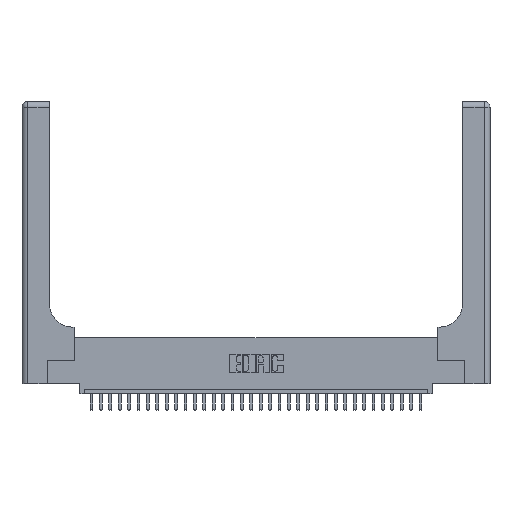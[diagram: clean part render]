
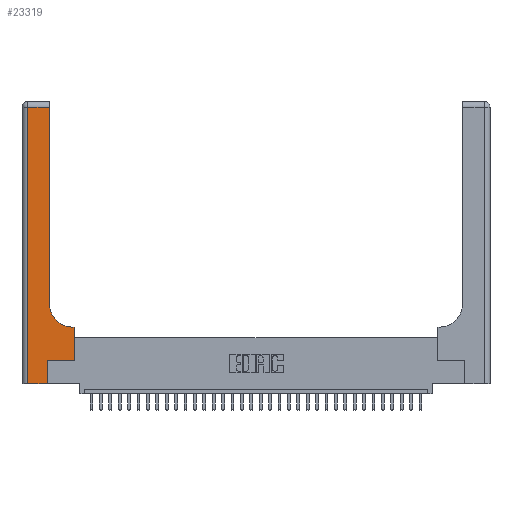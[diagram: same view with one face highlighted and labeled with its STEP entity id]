
A CAD part, top view. The second image highlights one B-rep face of the part: STEP entity #23319.
In plain terms, the highlighted planar face has unit normal (0, 0, 1).
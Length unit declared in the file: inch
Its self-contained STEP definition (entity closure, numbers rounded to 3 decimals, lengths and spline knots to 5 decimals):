
#301 = CARTESIAN_POINT ( 'NONE',  ( 0.06, 0., 0.37 ) ) ;
#767 = VECTOR ( 'NONE', #25287, 39.37008 ) ;
#1210 = CARTESIAN_POINT ( 'NONE',  ( 0.269, 0., 0.37 ) ) ;
#1386 = ORIENTED_EDGE ( 'NONE', *, *, #9491, .T. ) ;
#1639 = ORIENTED_EDGE ( 'NONE', *, *, #12392, .T. ) ;
#2786 = VERTEX_POINT ( 'NONE', #31323 ) ;
#3208 = CARTESIAN_POINT ( 'NONE',  ( 0.269, 0.25, 0.37 ) ) ;
#3319 = EDGE_CURVE ( 'NONE', #9044, #29370, #5518, .T. ) ;
#3731 = ORIENTED_EDGE ( 'NONE', *, *, #3319, .T. ) ;
#4740 = CARTESIAN_POINT ( 'NONE',  ( 0.5585, 0.6, 0.37 ) ) ;
#4770 = DIRECTION ( 'NONE',  ( 0., -1., 0. ) ) ;
#5312 = EDGE_CURVE ( 'NONE', #5352, #24309, #23494, .T. ) ;
#5352 = VERTEX_POINT ( 'NONE', #1210 ) ;
#5518 = LINE ( 'NONE', #20309, #29640 ) ;
#5809 = DIRECTION ( 'NONE',  ( 1., 0., 0. ) ) ;
#6129 = LINE ( 'NONE', #3208, #24587 ) ;
#6761 = VECTOR ( 'NONE', #26643, 39.37008 ) ;
#7242 = CARTESIAN_POINT ( 'NONE',  ( 0.5585, 0.25, 0.37 ) ) ;
#7351 = DIRECTION ( 'NONE',  ( 0., 0., -1. ) ) ;
#7523 = CARTESIAN_POINT ( 'NONE',  ( 0.269, 0.25, 0.37 ) ) ;
#7587 = EDGE_CURVE ( 'NONE', #28732, #2786, #20780, .T. ) ;
#7592 = LINE ( 'NONE', #20160, #767 ) ;
#8343 = ORIENTED_EDGE ( 'NONE', *, *, #32940, .T. ) ;
#8374 = CARTESIAN_POINT ( 'NONE',  ( 0., 3., 0.37 ) ) ;
#8383 = VERTEX_POINT ( 'NONE', #4740 ) ;
#8498 = ORIENTED_EDGE ( 'NONE', *, *, #11908, .T. ) ;
#8546 = CARTESIAN_POINT ( 'NONE',  ( 0.2915, 0.6, 0.37 ) ) ;
#8710 = DIRECTION ( 'NONE',  ( -1., 0., 0. ) ) ;
#9044 = VERTEX_POINT ( 'NONE', #19348 ) ;
#9491 = EDGE_CURVE ( 'NONE', #29370, #5352, #13828, .T. ) ;
#9790 = FACE_OUTER_BOUND ( 'NONE', #30020, .T. ) ;
#10191 = VECTOR ( 'NONE', #12410, 39.37008 ) ;
#10947 = DIRECTION ( 'NONE',  ( -1., 0., 0. ) ) ;
#11908 = EDGE_CURVE ( 'NONE', #2786, #16672, #7592, .T. ) ;
#12227 = LINE ( 'NONE', #16707, #14230 ) ;
#12392 = EDGE_CURVE ( 'NONE', #8383, #28732, #12775, .T. ) ;
#12410 = DIRECTION ( 'NONE',  ( 0., 1., 0. ) ) ;
#12775 = LINE ( 'NONE', #8546, #6761 ) ;
#12814 = DIRECTION ( 'NONE',  ( 0., 1., 0. ) ) ;
#12843 = CARTESIAN_POINT ( 'NONE',  ( 0.2915, 2.94, 0.37 ) ) ;
#13432 = DIRECTION ( 'NONE',  ( 0., 0., -1. ) ) ;
#13496 = CARTESIAN_POINT ( 'NONE',  ( 0., 0., 0.37 ) ) ;
#13828 = LINE ( 'NONE', #13496, #30327 ) ;
#14230 = VECTOR ( 'NONE', #8710, 39.37008 ) ;
#16614 = EDGE_CURVE ( 'NONE', #30853, #8383, #32746, .T. ) ;
#16672 = VERTEX_POINT ( 'NONE', #12843 ) ;
#16707 = CARTESIAN_POINT ( 'NONE',  ( 0., 2.94, 0.37 ) ) ;
#17613 = DIRECTION ( 'NONE',  ( 1., 0., 0. ) ) ;
#19348 = CARTESIAN_POINT ( 'NONE',  ( 0.06, 2.94, 0.37 ) ) ;
#20160 = CARTESIAN_POINT ( 'NONE',  ( 0.2915, 3., 0.37 ) ) ;
#20309 = CARTESIAN_POINT ( 'NONE',  ( 0.06, 3., 0.37 ) ) ;
#20780 = CIRCLE ( 'NONE', #29693, 0.25 ) ;
#21849 = CARTESIAN_POINT ( 'NONE',  ( 0.5585, 0.25, 0.37 ) ) ;
#22110 = ORIENTED_EDGE ( 'NONE', *, *, #5312, .T. ) ;
#22791 = CARTESIAN_POINT ( 'NONE',  ( 0.5415, 0.85, 0.37 ) ) ;
#22849 = ORIENTED_EDGE ( 'NONE', *, *, #16614, .T. ) ;
#23319 = ADVANCED_FACE ( 'NONE', ( #9790 ), #26449, .F. ) ;
#23471 = EDGE_CURVE ( 'NONE', #16672, #9044, #12227, .T. ) ;
#23494 = LINE ( 'NONE', #28543, #29082 ) ;
#24309 = VERTEX_POINT ( 'NONE', #7523 ) ;
#24587 = VECTOR ( 'NONE', #5809, 39.37008 ) ;
#25287 = DIRECTION ( 'NONE',  ( 0., 1., 0. ) ) ;
#26406 = DIRECTION ( 'NONE',  ( 1., 0., 0. ) ) ;
#26449 = PLANE ( 'NONE',  #30719 ) ;
#26643 = DIRECTION ( 'NONE',  ( -1., 0., 0. ) ) ;
#28543 = CARTESIAN_POINT ( 'NONE',  ( 0.269, 0., 0.37 ) ) ;
#28732 = VERTEX_POINT ( 'NONE', #31387 ) ;
#29082 = VECTOR ( 'NONE', #12814, 39.37008 ) ;
#29370 = VERTEX_POINT ( 'NONE', #301 ) ;
#29640 = VECTOR ( 'NONE', #4770, 39.37008 ) ;
#29693 = AXIS2_PLACEMENT_3D ( 'NONE', #22791, #7351, #17613 ) ;
#29772 = ORIENTED_EDGE ( 'NONE', *, *, #23471, .T. ) ;
#30020 = EDGE_LOOP ( 'NONE', ( #8498, #29772, #3731, #1386, #22110, #8343, #22849, #1639, #31148 ) ) ;
#30327 = VECTOR ( 'NONE', #26406, 39.37008 ) ;
#30719 = AXIS2_PLACEMENT_3D ( 'NONE', #8374, #13432, #10947 ) ;
#30853 = VERTEX_POINT ( 'NONE', #21849 ) ;
#31148 = ORIENTED_EDGE ( 'NONE', *, *, #7587, .T. ) ;
#31323 = CARTESIAN_POINT ( 'NONE',  ( 0.2915, 0.85, 0.37 ) ) ;
#31387 = CARTESIAN_POINT ( 'NONE',  ( 0.5415, 0.6, 0.37 ) ) ;
#32746 = LINE ( 'NONE', #7242, #10191 ) ;
#32940 = EDGE_CURVE ( 'NONE', #24309, #30853, #6129, .T. ) ;
